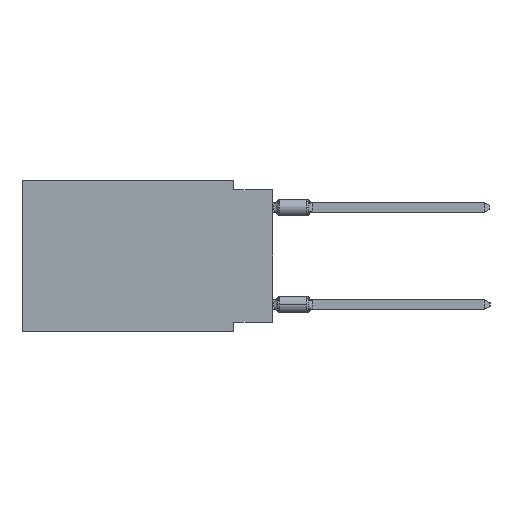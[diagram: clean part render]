
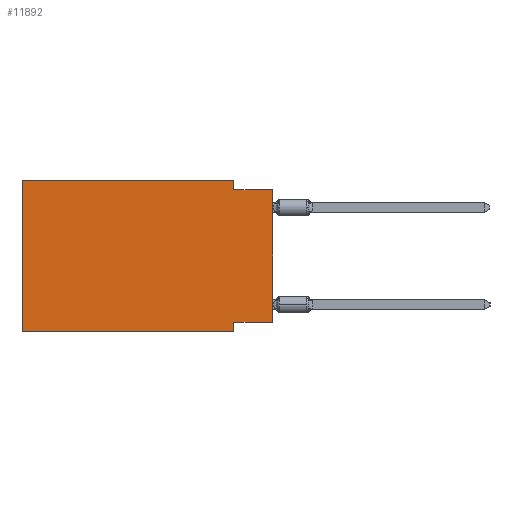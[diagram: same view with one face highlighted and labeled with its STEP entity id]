
A CAD part, left-side view. The second image highlights one B-rep face of the part: STEP entity #11892.
In plain terms, the highlighted planar face has unit normal (-1, 0, 0).
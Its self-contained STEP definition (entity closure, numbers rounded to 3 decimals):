
#1097 = LINE ( 'NONE', #40116, #4637 ) ;
#1452 = VERTEX_POINT ( 'NONE', #29406 ) ;
#2077 = EDGE_CURVE ( 'NONE', #61289, #1452, #1097, .T. ) ;
#3310 = ORIENTED_EDGE ( 'NONE', *, *, #47658, .F. ) ;
#4051 = PLANE ( 'NONE',  #27900 ) ;
#4194 = CARTESIAN_POINT ( 'NONE',  ( 0., 16.383, 0. ) ) ;
#4637 = VECTOR ( 'NONE', #40780, 1000. ) ;
#4693 = EDGE_CURVE ( 'NONE', #19032, #1452, #48743, .T. ) ;
#5244 = VERTEX_POINT ( 'NONE', #44068 ) ;
#7516 = LINE ( 'NONE', #33418, #20351 ) ;
#7857 = DIRECTION ( 'NONE',  ( 0., 1., 0. ) ) ;
#8965 = CARTESIAN_POINT ( 'NONE',  ( 0., 16.383, 0. ) ) ;
#9162 = VECTOR ( 'NONE', #29258, 1000. ) ;
#9857 = CARTESIAN_POINT ( 'NONE',  ( 0., 2.54, -0.635 ) ) ;
#11892 = ADVANCED_FACE ( 'NONE', ( #34210 ), #4051, .F. ) ;
#12750 = DIRECTION ( 'NONE',  ( 0., -1., 0. ) ) ;
#13077 = CARTESIAN_POINT ( 'NONE',  ( 0., 2.54, 0. ) ) ;
#13243 = EDGE_CURVE ( 'NONE', #30000, #25589, #58448, .T. ) ;
#15270 = CARTESIAN_POINT ( 'NONE',  ( 0., 0., -9.271 ) ) ;
#16419 = EDGE_CURVE ( 'NONE', #5244, #19032, #48166, .T. ) ;
#16964 = CARTESIAN_POINT ( 'NONE',  ( 0., 16.383, 0. ) ) ;
#19032 = VERTEX_POINT ( 'NONE', #9857 ) ;
#19567 = VECTOR ( 'NONE', #38890, 1000. ) ;
#19722 = VECTOR ( 'NONE', #32116, 1000. ) ;
#20351 = VECTOR ( 'NONE', #42940, 1000. ) ;
#23787 = LINE ( 'NONE', #43796, #24873 ) ;
#24390 = ORIENTED_EDGE ( 'NONE', *, *, #61256, .F. ) ;
#24873 = VECTOR ( 'NONE', #63776, 1000. ) ;
#25242 = EDGE_LOOP ( 'NONE', ( #27684, #60231, #26981, #24390, #3310, #62506, #52602, #54347 ) ) ;
#25589 = VERTEX_POINT ( 'NONE', #36405 ) ;
#26981 = ORIENTED_EDGE ( 'NONE', *, *, #16419, .F. ) ;
#27532 = VERTEX_POINT ( 'NONE', #44491 ) ;
#27684 = ORIENTED_EDGE ( 'NONE', *, *, #2077, .T. ) ;
#27900 = AXIS2_PLACEMENT_3D ( 'NONE', #8965, #63080, #39126 ) ;
#29258 = DIRECTION ( 'NONE',  ( 0., 0., -1. ) ) ;
#29406 = CARTESIAN_POINT ( 'NONE',  ( 0., 0., -0.635 ) ) ;
#30000 = VERTEX_POINT ( 'NONE', #33985 ) ;
#32116 = DIRECTION ( 'NONE',  ( 0., 0., -1. ) ) ;
#33418 = CARTESIAN_POINT ( 'NONE',  ( 0., 16.383, -9.906 ) ) ;
#33662 = CARTESIAN_POINT ( 'NONE',  ( 0., 0., -0.635 ) ) ;
#33985 = CARTESIAN_POINT ( 'NONE',  ( 0., 2.54, -9.271 ) ) ;
#34210 = FACE_OUTER_BOUND ( 'NONE', #25242, .T. ) ;
#36405 = CARTESIAN_POINT ( 'NONE',  ( 0., 2.54, -9.906 ) ) ;
#38890 = DIRECTION ( 'NONE',  ( 0., -1., 0. ) ) ;
#39126 = DIRECTION ( 'NONE',  ( 0., 0., -1. ) ) ;
#39913 = CARTESIAN_POINT ( 'NONE',  ( 0., 0., -9.271 ) ) ;
#40116 = CARTESIAN_POINT ( 'NONE',  ( 0., 0., 0. ) ) ;
#40780 = DIRECTION ( 'NONE',  ( 0., 0., 1. ) ) ;
#42940 = DIRECTION ( 'NONE',  ( 0., -1., 0. ) ) ;
#43796 = CARTESIAN_POINT ( 'NONE',  ( 0., 16.383, 0. ) ) ;
#44068 = CARTESIAN_POINT ( 'NONE',  ( 0., 2.54, 0. ) ) ;
#44337 = CARTESIAN_POINT ( 'NONE',  ( 0., 2.54, -9.906 ) ) ;
#44491 = CARTESIAN_POINT ( 'NONE',  ( 0., 16.383, -9.906 ) ) ;
#46766 = VECTOR ( 'NONE', #7857, 1000. ) ;
#47658 = EDGE_CURVE ( 'NONE', #27532, #61451, #23787, .T. ) ;
#48166 = LINE ( 'NONE', #13077, #19722 ) ;
#48743 = LINE ( 'NONE', #33662, #19567 ) ;
#48805 = LINE ( 'NONE', #4194, #49166 ) ;
#49166 = VECTOR ( 'NONE', #12750, 1000. ) ;
#52602 = ORIENTED_EDGE ( 'NONE', *, *, #13243, .F. ) ;
#53565 = EDGE_CURVE ( 'NONE', #27532, #25589, #7516, .T. ) ;
#54347 = ORIENTED_EDGE ( 'NONE', *, *, #55336, .F. ) ;
#55336 = EDGE_CURVE ( 'NONE', #61289, #30000, #58026, .T. ) ;
#58026 = LINE ( 'NONE', #15270, #46766 ) ;
#58448 = LINE ( 'NONE', #44337, #9162 ) ;
#60231 = ORIENTED_EDGE ( 'NONE', *, *, #4693, .F. ) ;
#61256 = EDGE_CURVE ( 'NONE', #61451, #5244, #48805, .T. ) ;
#61289 = VERTEX_POINT ( 'NONE', #39913 ) ;
#61451 = VERTEX_POINT ( 'NONE', #16964 ) ;
#62506 = ORIENTED_EDGE ( 'NONE', *, *, #53565, .T. ) ;
#63080 = DIRECTION ( 'NONE',  ( 1., 0., 0. ) ) ;
#63776 = DIRECTION ( 'NONE',  ( 0., 0., 1. ) ) ;
